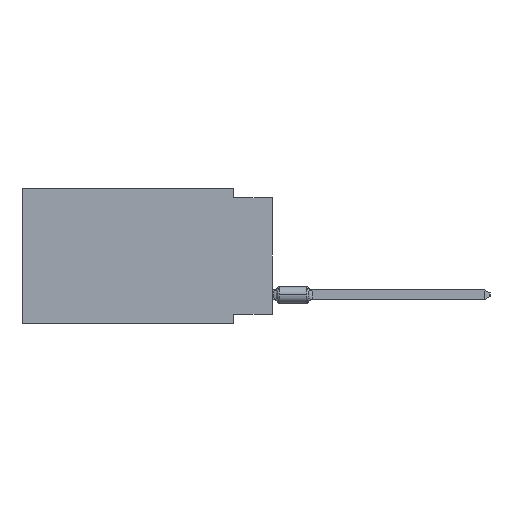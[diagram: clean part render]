
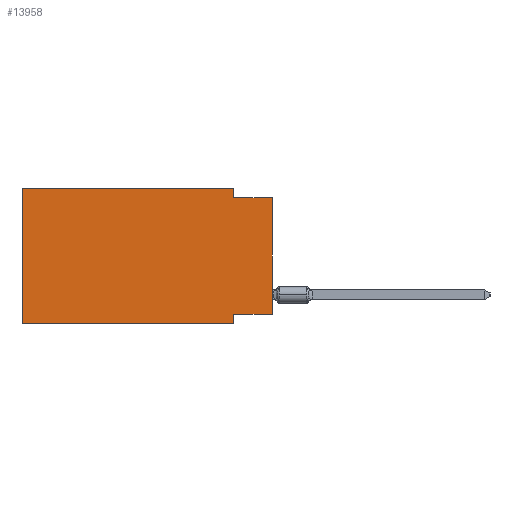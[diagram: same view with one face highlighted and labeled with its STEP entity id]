
A CAD part, left-side view. The second image highlights one B-rep face of the part: STEP entity #13958.
In plain terms, the highlighted planar face has unit normal (-1, 0, 0).
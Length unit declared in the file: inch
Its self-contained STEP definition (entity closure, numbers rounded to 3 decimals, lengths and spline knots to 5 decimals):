
#104 = DIRECTION ( 'NONE',  ( 0., 0., -1. ) ) ;
#814 = CARTESIAN_POINT ( 'NONE',  ( 0., 0.645, 0. ) ) ;
#983 = LINE ( 'NONE', #19351, #42440 ) ;
#1481 = VECTOR ( 'NONE', #9581, 39.37008 ) ;
#1889 = CARTESIAN_POINT ( 'NONE',  ( 0., 0.645, 0. ) ) ;
#2841 = VECTOR ( 'NONE', #25972, 39.37008 ) ;
#3795 = DIRECTION ( 'NONE',  ( 0., -1., 0. ) ) ;
#3914 = CARTESIAN_POINT ( 'NONE',  ( 0., 0.1, -0.35 ) ) ;
#4035 = LINE ( 'NONE', #19175, #9722 ) ;
#5047 = CARTESIAN_POINT ( 'NONE',  ( 0., 0.645, 0. ) ) ;
#5313 = ORIENTED_EDGE ( 'NONE', *, *, #19925, .F. ) ;
#5748 = ORIENTED_EDGE ( 'NONE', *, *, #36631, .F. ) ;
#5875 = VERTEX_POINT ( 'NONE', #47441 ) ;
#8447 = VERTEX_POINT ( 'NONE', #3914 ) ;
#9581 = DIRECTION ( 'NONE',  ( 0., 0., 1. ) ) ;
#9722 = VECTOR ( 'NONE', #3795, 39.37008 ) ;
#9920 = CARTESIAN_POINT ( 'NONE',  ( 0., 0.1, -0.35 ) ) ;
#9947 = VECTOR ( 'NONE', #14025, 39.37008 ) ;
#10943 = ORIENTED_EDGE ( 'NONE', *, *, #12448, .T. ) ;
#11277 = LINE ( 'NONE', #21694, #9947 ) ;
#12448 = EDGE_CURVE ( 'NONE', #20100, #38329, #42866, .T. ) ;
#12471 = AXIS2_PLACEMENT_3D ( 'NONE', #5047, #34070, #104 ) ;
#12495 = FACE_OUTER_BOUND ( 'NONE', #41973, .T. ) ;
#12617 = DIRECTION ( 'NONE',  ( 0., 0., 1. ) ) ;
#13123 = VECTOR ( 'NONE', #12617, 39.37008 ) ;
#13958 = ADVANCED_FACE ( 'NONE', ( #12495 ), #39016, .F. ) ;
#14025 = DIRECTION ( 'NONE',  ( 0., 1., 0. ) ) ;
#14891 = VERTEX_POINT ( 'NONE', #35664 ) ;
#15565 = ORIENTED_EDGE ( 'NONE', *, *, #36085, .F. ) ;
#16052 = EDGE_CURVE ( 'NONE', #33089, #48732, #40634, .T. ) ;
#17070 = EDGE_CURVE ( 'NONE', #14891, #33089, #36109, .T. ) ;
#18349 = ORIENTED_EDGE ( 'NONE', *, *, #17070, .F. ) ;
#19059 = ORIENTED_EDGE ( 'NONE', *, *, #16052, .F. ) ;
#19175 = CARTESIAN_POINT ( 'NONE',  ( 0., 0.645, -0.35 ) ) ;
#19351 = CARTESIAN_POINT ( 'NONE',  ( 0., 0.1, 0. ) ) ;
#19925 = EDGE_CURVE ( 'NONE', #20100, #41178, #11277, .T. ) ;
#20100 = VERTEX_POINT ( 'NONE', #34580 ) ;
#21132 = VECTOR ( 'NONE', #25290, 39.37008 ) ;
#21273 = EDGE_CURVE ( 'NONE', #41178, #8447, #25518, .T. ) ;
#21694 = CARTESIAN_POINT ( 'NONE',  ( 0., 0., -0.325 ) ) ;
#23282 = DIRECTION ( 'NONE',  ( 0., 0., -1. ) ) ;
#24828 = CARTESIAN_POINT ( 'NONE',  ( 0., 0., -0.025 ) ) ;
#25244 = CARTESIAN_POINT ( 'NONE',  ( 0., 0., -0.025 ) ) ;
#25266 = DIRECTION ( 'NONE',  ( 0., -1., 0. ) ) ;
#25290 = DIRECTION ( 'NONE',  ( 0., 0., -1. ) ) ;
#25518 = LINE ( 'NONE', #9920, #21132 ) ;
#25717 = LINE ( 'NONE', #25244, #2841 ) ;
#25972 = DIRECTION ( 'NONE',  ( 0., -1., 0. ) ) ;
#32918 = CARTESIAN_POINT ( 'NONE',  ( 0., 0.1, 0. ) ) ;
#33018 = EDGE_CURVE ( 'NONE', #14891, #8447, #4035, .T. ) ;
#33089 = VERTEX_POINT ( 'NONE', #814 ) ;
#34070 = DIRECTION ( 'NONE',  ( 1., 0., 0. ) ) ;
#34580 = CARTESIAN_POINT ( 'NONE',  ( 0., 0., -0.325 ) ) ;
#35552 = ORIENTED_EDGE ( 'NONE', *, *, #33018, .T. ) ;
#35664 = CARTESIAN_POINT ( 'NONE',  ( 0., 0.645, -0.35 ) ) ;
#36085 = EDGE_CURVE ( 'NONE', #48732, #5875, #983, .T. ) ;
#36109 = LINE ( 'NONE', #1889, #1481 ) ;
#36631 = EDGE_CURVE ( 'NONE', #5875, #38329, #25717, .T. ) ;
#37839 = VECTOR ( 'NONE', #25266, 39.37008 ) ;
#38329 = VERTEX_POINT ( 'NONE', #24828 ) ;
#39016 = PLANE ( 'NONE',  #12471 ) ;
#40634 = LINE ( 'NONE', #48087, #37839 ) ;
#41178 = VERTEX_POINT ( 'NONE', #46732 ) ;
#41973 = EDGE_LOOP ( 'NONE', ( #10943, #5748, #15565, #19059, #18349, #35552, #48431, #5313 ) ) ;
#42440 = VECTOR ( 'NONE', #23282, 39.37008 ) ;
#42866 = LINE ( 'NONE', #47307, #13123 ) ;
#46732 = CARTESIAN_POINT ( 'NONE',  ( 0., 0.1, -0.325 ) ) ;
#47307 = CARTESIAN_POINT ( 'NONE',  ( 0., 0., 0. ) ) ;
#47441 = CARTESIAN_POINT ( 'NONE',  ( 0., 0.1, -0.025 ) ) ;
#48087 = CARTESIAN_POINT ( 'NONE',  ( 0., 0.645, 0. ) ) ;
#48431 = ORIENTED_EDGE ( 'NONE', *, *, #21273, .F. ) ;
#48732 = VERTEX_POINT ( 'NONE', #32918 ) ;
